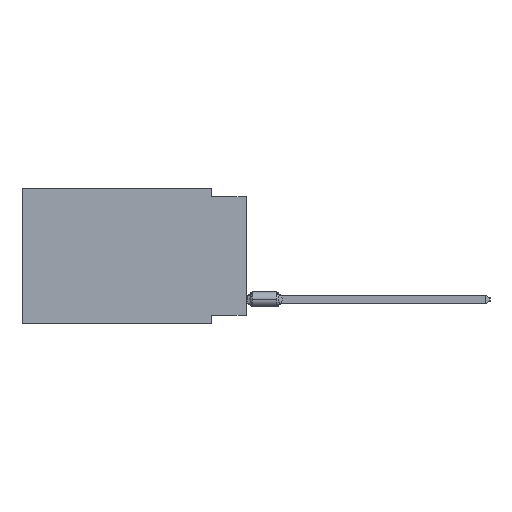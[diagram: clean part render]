
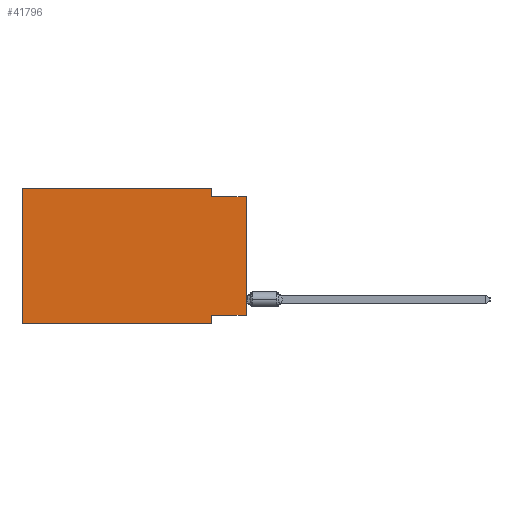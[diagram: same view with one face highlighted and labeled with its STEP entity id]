
A CAD part, left-side view. The second image highlights one B-rep face of the part: STEP entity #41796.
In plain terms, the highlighted planar face has unit normal (-1, 0, 0).
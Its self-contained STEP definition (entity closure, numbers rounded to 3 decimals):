
#138 = VERTEX_POINT ( 'NONE', #49909 ) ;
#733 = CARTESIAN_POINT ( 'NONE',  ( 0., 16.383, 0. ) ) ;
#1637 = ORIENTED_EDGE ( 'NONE', *, *, #8260, .F. ) ;
#1829 = VERTEX_POINT ( 'NONE', #35310 ) ;
#3659 = EDGE_CURVE ( 'NONE', #13446, #30042, #36111, .T. ) ;
#4016 = CARTESIAN_POINT ( 'NONE',  ( 0., 16.383, 0. ) ) ;
#4387 = LINE ( 'NONE', #23112, #27053 ) ;
#4596 = ORIENTED_EDGE ( 'NONE', *, *, #11103, .F. ) ;
#5779 = VERTEX_POINT ( 'NONE', #59673 ) ;
#5886 = AXIS2_PLACEMENT_3D ( 'NONE', #4016, #42604, #12631 ) ;
#6855 = ORIENTED_EDGE ( 'NONE', *, *, #50760, .T. ) ;
#7370 = ORIENTED_EDGE ( 'NONE', *, *, #20960, .T. ) ;
#7582 = LINE ( 'NONE', #55183, #28626 ) ;
#7771 = VECTOR ( 'NONE', #49969, 1000. ) ;
#8260 = EDGE_CURVE ( 'NONE', #138, #48043, #50265, .T. ) ;
#8930 = CARTESIAN_POINT ( 'NONE',  ( 0., 2.54, -0.635 ) ) ;
#11103 = EDGE_CURVE ( 'NONE', #16396, #5779, #57018, .T. ) ;
#11738 = LINE ( 'NONE', #22163, #38198 ) ;
#12631 = DIRECTION ( 'NONE',  ( 0., 0., -1. ) ) ;
#12979 = DIRECTION ( 'NONE',  ( 0., -1., 0. ) ) ;
#13116 = DIRECTION ( 'NONE',  ( 0., 0., -1. ) ) ;
#13446 = VERTEX_POINT ( 'NONE', #20524 ) ;
#14855 = ORIENTED_EDGE ( 'NONE', *, *, #34324, .F. ) ;
#14931 = CARTESIAN_POINT ( 'NONE',  ( 0., 0., -0.635 ) ) ;
#16396 = VERTEX_POINT ( 'NONE', #8930 ) ;
#19662 = CARTESIAN_POINT ( 'NONE',  ( 0., 16.383, 0. ) ) ;
#20524 = CARTESIAN_POINT ( 'NONE',  ( 0., 16.383, -9.906 ) ) ;
#20960 = EDGE_CURVE ( 'NONE', #13446, #1829, #49815, .T. ) ;
#22163 = CARTESIAN_POINT ( 'NONE',  ( 0., 2.54, 0. ) ) ;
#22922 = CARTESIAN_POINT ( 'NONE',  ( 0., 16.383, 0. ) ) ;
#23112 = CARTESIAN_POINT ( 'NONE',  ( 0., 0., 0. ) ) ;
#23876 = FACE_OUTER_BOUND ( 'NONE', #25407, .T. ) ;
#23956 = DIRECTION ( 'NONE',  ( 0., -1., 0. ) ) ;
#24325 = CARTESIAN_POINT ( 'NONE',  ( 0., 2.54, -9.271 ) ) ;
#25219 = VECTOR ( 'NONE', #12979, 1000. ) ;
#25407 = EDGE_LOOP ( 'NONE', ( #6855, #4596, #52103, #58445, #49802, #7370, #14855, #1637 ) ) ;
#27053 = VECTOR ( 'NONE', #41826, 1000. ) ;
#28475 = PLANE ( 'NONE',  #5886 ) ;
#28626 = VECTOR ( 'NONE', #13116, 1000. ) ;
#28668 = VECTOR ( 'NONE', #51469, 1000. ) ;
#30042 = VERTEX_POINT ( 'NONE', #733 ) ;
#34324 = EDGE_CURVE ( 'NONE', #48043, #1829, #7582, .T. ) ;
#35310 = CARTESIAN_POINT ( 'NONE',  ( 0., 2.54, -9.906 ) ) ;
#36111 = LINE ( 'NONE', #22922, #58021 ) ;
#36442 = CARTESIAN_POINT ( 'NONE',  ( 0., 0., -9.271 ) ) ;
#38198 = VECTOR ( 'NONE', #50085, 1000. ) ;
#41796 = ADVANCED_FACE ( 'NONE', ( #23876 ), #28475, .F. ) ;
#41826 = DIRECTION ( 'NONE',  ( 0., 0., 1. ) ) ;
#42604 = DIRECTION ( 'NONE',  ( 1., 0., 0. ) ) ;
#43353 = EDGE_CURVE ( 'NONE', #51945, #16396, #11738, .T. ) ;
#44028 = EDGE_CURVE ( 'NONE', #30042, #51945, #47278, .T. ) ;
#44317 = CARTESIAN_POINT ( 'NONE',  ( 0., 2.54, 0. ) ) ;
#47278 = LINE ( 'NONE', #19662, #54935 ) ;
#48043 = VERTEX_POINT ( 'NONE', #24325 ) ;
#49802 = ORIENTED_EDGE ( 'NONE', *, *, #3659, .F. ) ;
#49815 = LINE ( 'NONE', #60288, #25219 ) ;
#49909 = CARTESIAN_POINT ( 'NONE',  ( 0., 0., -9.271 ) ) ;
#49969 = DIRECTION ( 'NONE',  ( 0., 1., 0. ) ) ;
#50085 = DIRECTION ( 'NONE',  ( 0., 0., -1. ) ) ;
#50265 = LINE ( 'NONE', #36442, #7771 ) ;
#50760 = EDGE_CURVE ( 'NONE', #138, #5779, #4387, .T. ) ;
#51469 = DIRECTION ( 'NONE',  ( 0., -1., 0. ) ) ;
#51945 = VERTEX_POINT ( 'NONE', #44317 ) ;
#52103 = ORIENTED_EDGE ( 'NONE', *, *, #43353, .F. ) ;
#54935 = VECTOR ( 'NONE', #23956, 1000. ) ;
#55183 = CARTESIAN_POINT ( 'NONE',  ( 0., 2.54, -9.906 ) ) ;
#57018 = LINE ( 'NONE', #14931, #28668 ) ;
#58021 = VECTOR ( 'NONE', #59193, 1000. ) ;
#58445 = ORIENTED_EDGE ( 'NONE', *, *, #44028, .F. ) ;
#59193 = DIRECTION ( 'NONE',  ( 0., 0., 1. ) ) ;
#59673 = CARTESIAN_POINT ( 'NONE',  ( 0., 0., -0.635 ) ) ;
#60288 = CARTESIAN_POINT ( 'NONE',  ( 0., 16.383, -9.906 ) ) ;
